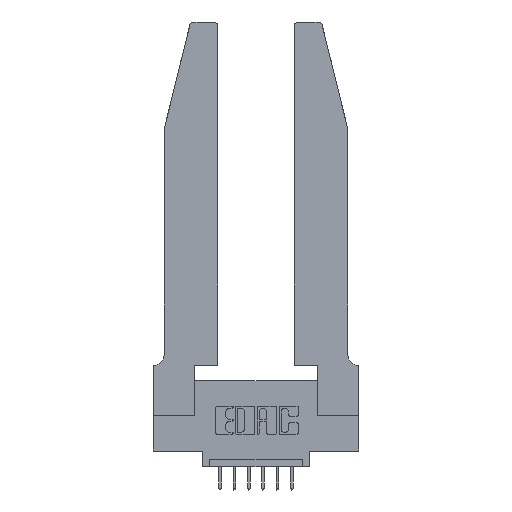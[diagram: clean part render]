
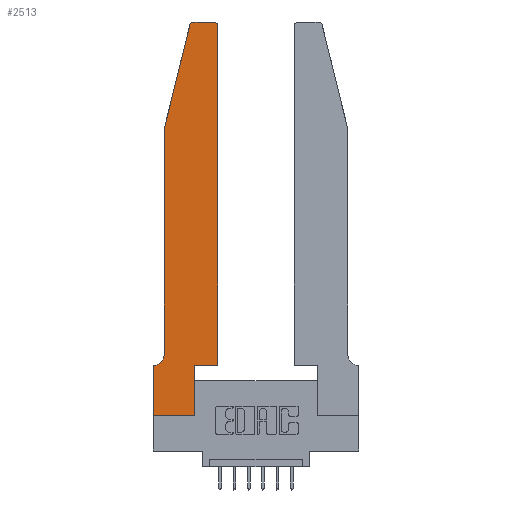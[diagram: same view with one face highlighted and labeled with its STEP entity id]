
A CAD part, top view. The second image highlights one B-rep face of the part: STEP entity #2513.
In plain terms, the highlighted planar face has unit normal (0, 0, 1).
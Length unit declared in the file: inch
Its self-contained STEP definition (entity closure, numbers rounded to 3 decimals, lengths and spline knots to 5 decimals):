
#12 = LINE ( 'NONE', #3705, #7824 ) ;
#399 = EDGE_CURVE ( 'NONE', #1019, #10248, #5087, .T. ) ;
#454 = CARTESIAN_POINT ( 'NONE',  ( 0., 0., 0.37 ) ) ;
#602 = EDGE_CURVE ( 'NONE', #12680, #2958, #13911, .T. ) ;
#704 = ORIENTED_EDGE ( 'NONE', *, *, #11186, .T. ) ;
#893 = DIRECTION ( 'NONE',  ( 0., -1., 0. ) ) ;
#934 = CARTESIAN_POINT ( 'NONE',  ( 0.4505, 2.72, 0.37 ) ) ;
#1019 = VERTEX_POINT ( 'NONE', #7313 ) ;
#1149 = LINE ( 'NONE', #6357, #9653 ) ;
#1154 = CARTESIAN_POINT ( 'NONE',  ( 0.0755, 2., 0.37 ) ) ;
#1220 = EDGE_CURVE ( 'NONE', #10248, #6199, #9770, .T. ) ;
#1276 = CARTESIAN_POINT ( 'NONE',  ( 0.4205, 2.75, 0.37 ) ) ;
#1386 = AXIS2_PLACEMENT_3D ( 'NONE', #8697, #10816, #14280 ) ;
#1570 = VECTOR ( 'NONE', #8378, 39.37008 ) ;
#1731 = CARTESIAN_POINT ( 'NONE',  ( 0.0055, 0.35, 0.37 ) ) ;
#2187 = EDGE_CURVE ( 'NONE', #5735, #7817, #5753, .T. ) ;
#2189 = AXIS2_PLACEMENT_3D ( 'NONE', #5998, #12783, #11764 ) ;
#2261 = CIRCLE ( 'NONE', #2189, 0.03 ) ;
#2310 = ORIENTED_EDGE ( 'NONE', *, *, #602, .T. ) ;
#2513 = ADVANCED_FACE ( 'NONE', ( #10424 ), #7484, .T. ) ;
#2568 = DIRECTION ( 'NONE',  ( -1., 0., 0. ) ) ;
#2958 = VERTEX_POINT ( 'NONE', #12407 ) ;
#3060 = EDGE_CURVE ( 'NONE', #2958, #10181, #12, .T. ) ;
#3153 = CARTESIAN_POINT ( 'NONE',  ( 0.4505, 0.35, 0.37 ) ) ;
#3230 = VECTOR ( 'NONE', #13857, 39.37008 ) ;
#3308 = AXIS2_PLACEMENT_3D ( 'NONE', #11548, #11709, #9414 ) ;
#3443 = ORIENTED_EDGE ( 'NONE', *, *, #399, .T. ) ;
#3527 = ORIENTED_EDGE ( 'NONE', *, *, #6058, .T. ) ;
#3616 = VECTOR ( 'NONE', #2568, 39.37008 ) ;
#3705 = CARTESIAN_POINT ( 'NONE',  ( 0.4505, 0.35, 0.37 ) ) ;
#3709 = ORIENTED_EDGE ( 'NONE', *, *, #3744, .T. ) ;
#3710 = VERTEX_POINT ( 'NONE', #7236 ) ;
#3744 = EDGE_CURVE ( 'NONE', #3710, #12680, #10546, .T. ) ;
#3752 = DIRECTION ( 'NONE',  ( 0., 1., 0. ) ) ;
#3755 = VERTEX_POINT ( 'NONE', #934 ) ;
#4069 = ORIENTED_EDGE ( 'NONE', *, *, #4165, .T. ) ;
#4145 = DIRECTION ( 'NONE',  ( 1., 0., 0. ) ) ;
#4165 = EDGE_CURVE ( 'NONE', #11093, #5735, #8511, .T. ) ;
#4394 = VECTOR ( 'NONE', #3752, 39.37008 ) ;
#4545 = CARTESIAN_POINT ( 'NONE',  ( 0.4505, 0.35, 0.37 ) ) ;
#4742 = VERTEX_POINT ( 'NONE', #1154 ) ;
#4953 = EDGE_CURVE ( 'NONE', #10181, #3755, #9681, .T. ) ;
#5087 = CIRCLE ( 'NONE', #3308, 0.07 ) ;
#5735 = VERTEX_POINT ( 'NONE', #7033 ) ;
#5753 = CIRCLE ( 'NONE', #11030, 0.03 ) ;
#5998 = CARTESIAN_POINT ( 'NONE',  ( 0.4205, 2.72, 0.37 ) ) ;
#6058 = EDGE_CURVE ( 'NONE', #6199, #3710, #12576, .T. ) ;
#6174 = LINE ( 'NONE', #12663, #3230 ) ;
#6199 = VERTEX_POINT ( 'NONE', #6960 ) ;
#6357 = CARTESIAN_POINT ( 'NONE',  ( 0.0755, 2., 0.37 ) ) ;
#6571 = ORIENTED_EDGE ( 'NONE', *, *, #9230, .T. ) ;
#6960 = CARTESIAN_POINT ( 'NONE',  ( 0., 0.35, 0.37 ) ) ;
#7033 = CARTESIAN_POINT ( 'NONE',  ( 0.284, 2.75, 0.37 ) ) ;
#7236 = CARTESIAN_POINT ( 'NONE',  ( 0., 0., 0.37 ) ) ;
#7313 = CARTESIAN_POINT ( 'NONE',  ( 0.0755, 0.42, 0.37 ) ) ;
#7438 = ORIENTED_EDGE ( 'NONE', *, *, #1220, .T. ) ;
#7467 = ORIENTED_EDGE ( 'NONE', *, *, #2187, .T. ) ;
#7468 = ORIENTED_EDGE ( 'NONE', *, *, #11722, .T. ) ;
#7484 = PLANE ( 'NONE',  #1386 ) ;
#7817 = VERTEX_POINT ( 'NONE', #13534 ) ;
#7824 = VECTOR ( 'NONE', #9199, 39.37008 ) ;
#8239 = VECTOR ( 'NONE', #14344, 39.37008 ) ;
#8378 = DIRECTION ( 'NONE',  ( 1., 0., 0. ) ) ;
#8511 = LINE ( 'NONE', #10402, #3616 ) ;
#8697 = CARTESIAN_POINT ( 'NONE',  ( 0., 0.35, 0.37 ) ) ;
#9008 = CARTESIAN_POINT ( 'NONE',  ( 0.0755, 0.35, 0.37 ) ) ;
#9199 = DIRECTION ( 'NONE',  ( 1., 0., 0. ) ) ;
#9230 = EDGE_CURVE ( 'NONE', #3755, #11093, #2261, .T. ) ;
#9414 = DIRECTION ( 'NONE',  ( -1., 0., 0. ) ) ;
#9653 = VECTOR ( 'NONE', #893, 39.37008 ) ;
#9681 = LINE ( 'NONE', #3153, #13467 ) ;
#9770 = LINE ( 'NONE', #9008, #8239 ) ;
#10181 = VERTEX_POINT ( 'NONE', #4545 ) ;
#10248 = VERTEX_POINT ( 'NONE', #1731 ) ;
#10402 = CARTESIAN_POINT ( 'NONE',  ( 0.2605, 2.75, 0.37 ) ) ;
#10424 = FACE_OUTER_BOUND ( 'NONE', #11836, .T. ) ;
#10546 = LINE ( 'NONE', #11603, #1570 ) ;
#10614 = ORIENTED_EDGE ( 'NONE', *, *, #4953, .T. ) ;
#10816 = DIRECTION ( 'NONE',  ( 0., 0., 1. ) ) ;
#11030 = AXIS2_PLACEMENT_3D ( 'NONE', #14157, #13142, #4145 ) ;
#11093 = VERTEX_POINT ( 'NONE', #1276 ) ;
#11186 = EDGE_CURVE ( 'NONE', #7817, #4742, #6174, .T. ) ;
#11548 = CARTESIAN_POINT ( 'NONE',  ( 0.0055, 0.42, 0.37 ) ) ;
#11603 = CARTESIAN_POINT ( 'NONE',  ( 0., 0., 0.37 ) ) ;
#11618 = CARTESIAN_POINT ( 'NONE',  ( 0.2865, 0.35, 0.37 ) ) ;
#11646 = CARTESIAN_POINT ( 'NONE',  ( 0.2865, 0., 0.37 ) ) ;
#11709 = DIRECTION ( 'NONE',  ( 0., 0., -1. ) ) ;
#11722 = EDGE_CURVE ( 'NONE', #4742, #1019, #1149, .T. ) ;
#11764 = DIRECTION ( 'NONE',  ( 1., 0., 0. ) ) ;
#11836 = EDGE_LOOP ( 'NONE', ( #4069, #7467, #704, #7468, #3443, #7438, #3527, #3709, #2310, #13999, #10614, #6571 ) ) ;
#12407 = CARTESIAN_POINT ( 'NONE',  ( 0.2865, 0.35, 0.37 ) ) ;
#12576 = LINE ( 'NONE', #454, #12744 ) ;
#12663 = CARTESIAN_POINT ( 'NONE',  ( 0.0755, 2., 0.37 ) ) ;
#12680 = VERTEX_POINT ( 'NONE', #11646 ) ;
#12744 = VECTOR ( 'NONE', #13220, 39.37008 ) ;
#12783 = DIRECTION ( 'NONE',  ( 0., 0., 1. ) ) ;
#13142 = DIRECTION ( 'NONE',  ( 0., 0., 1. ) ) ;
#13220 = DIRECTION ( 'NONE',  ( 0., -1., 0. ) ) ;
#13467 = VECTOR ( 'NONE', #14147, 39.37008 ) ;
#13534 = CARTESIAN_POINT ( 'NONE',  ( 0.25487, 2.72718, 0.37 ) ) ;
#13857 = DIRECTION ( 'NONE',  ( -0.239, -0.971, 0. ) ) ;
#13911 = LINE ( 'NONE', #11618, #4394 ) ;
#13999 = ORIENTED_EDGE ( 'NONE', *, *, #3060, .T. ) ;
#14147 = DIRECTION ( 'NONE',  ( 0., 1., 0. ) ) ;
#14157 = CARTESIAN_POINT ( 'NONE',  ( 0.284, 2.72, 0.37 ) ) ;
#14280 = DIRECTION ( 'NONE',  ( 1., 0., 0. ) ) ;
#14344 = DIRECTION ( 'NONE',  ( -1., 0., 0. ) ) ;
